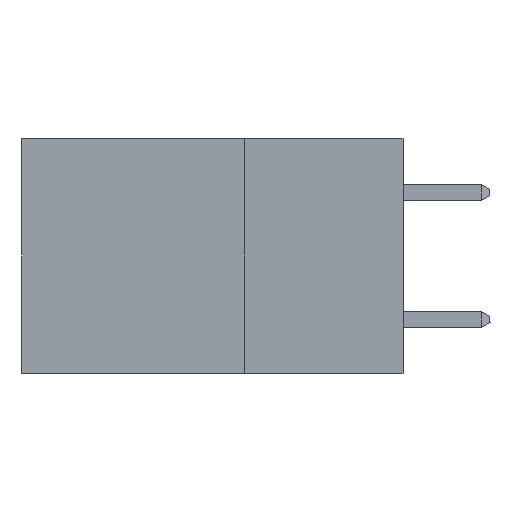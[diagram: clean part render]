
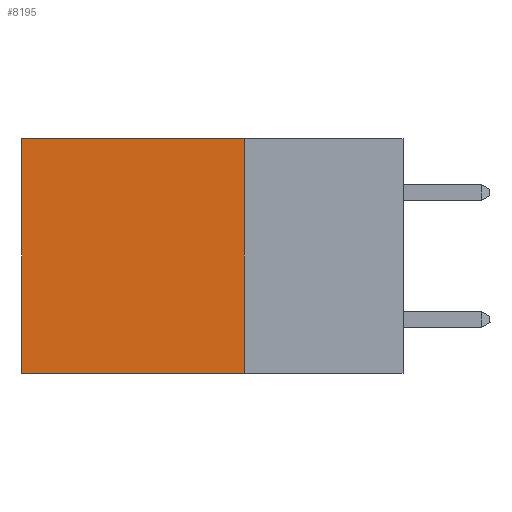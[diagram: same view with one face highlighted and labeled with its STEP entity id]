
A CAD part, left-side view. The second image highlights one B-rep face of the part: STEP entity #8195.
In plain terms, the highlighted planar face has unit normal (-1, 0, 0).
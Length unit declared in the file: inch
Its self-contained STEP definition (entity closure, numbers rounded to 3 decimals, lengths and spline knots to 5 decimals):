
#288 = LINE ( 'NONE', #4807, #12843 ) ;
#349 = CARTESIAN_POINT ( 'NONE',  ( 0.2875, 0.25, 0. ) ) ;
#1516 = DIRECTION ( 'NONE',  ( 0., 0., -1. ) ) ;
#1641 = LINE ( 'NONE', #9368, #4037 ) ;
#2207 = CARTESIAN_POINT ( 'NONE',  ( 0.2875, 0.25, 0. ) ) ;
#2463 = EDGE_CURVE ( 'NONE', #10971, #2933, #1641, .T. ) ;
#2933 = VERTEX_POINT ( 'NONE', #4851 ) ;
#3412 = DIRECTION ( 'NONE',  ( 1., 0., 0. ) ) ;
#3522 = FACE_OUTER_BOUND ( 'NONE', #11455, .T. ) ;
#4037 = VECTOR ( 'NONE', #1516, 39.37008 ) ;
#4088 = VERTEX_POINT ( 'NONE', #11445 ) ;
#4428 = LINE ( 'NONE', #11561, #7418 ) ;
#4807 = CARTESIAN_POINT ( 'NONE',  ( 0.2875, 0.25, -0.37 ) ) ;
#4851 = CARTESIAN_POINT ( 'NONE',  ( 0.2875, 0.25, -0.37 ) ) ;
#6516 = ORIENTED_EDGE ( 'NONE', *, *, #8967, .T. ) ;
#6589 = DIRECTION ( 'NONE',  ( 0., 0., -1. ) ) ;
#7290 = AXIS2_PLACEMENT_3D ( 'NONE', #2207, #3412, #12049 ) ;
#7418 = VECTOR ( 'NONE', #6589, 39.37008 ) ;
#7448 = CARTESIAN_POINT ( 'NONE',  ( 0.2875, 0.25, 0. ) ) ;
#7703 = LINE ( 'NONE', #349, #13649 ) ;
#8193 = ORIENTED_EDGE ( 'NONE', *, *, #9516, .F. ) ;
#8195 = ADVANCED_FACE ( 'NONE', ( #3522 ), #9686, .F. ) ;
#8201 = CARTESIAN_POINT ( 'NONE',  ( 0.2875, 0.6, 0. ) ) ;
#8801 = ORIENTED_EDGE ( 'NONE', *, *, #2463, .F. ) ;
#8962 = DIRECTION ( 'NONE',  ( 0., 1., 0. ) ) ;
#8967 = EDGE_CURVE ( 'NONE', #12378, #4088, #4428, .T. ) ;
#9130 = ORIENTED_EDGE ( 'NONE', *, *, #14373, .T. ) ;
#9368 = CARTESIAN_POINT ( 'NONE',  ( 0.2875, 0.25, 0. ) ) ;
#9516 = EDGE_CURVE ( 'NONE', #2933, #4088, #288, .T. ) ;
#9686 = PLANE ( 'NONE',  #7290 ) ;
#10971 = VERTEX_POINT ( 'NONE', #7448 ) ;
#11445 = CARTESIAN_POINT ( 'NONE',  ( 0.2875, 0.6, -0.37 ) ) ;
#11455 = EDGE_LOOP ( 'NONE', ( #6516, #8193, #8801, #9130 ) ) ;
#11561 = CARTESIAN_POINT ( 'NONE',  ( 0.2875, 0.6, 0. ) ) ;
#12049 = DIRECTION ( 'NONE',  ( 0., 0., -1. ) ) ;
#12242 = DIRECTION ( 'NONE',  ( 0., 1., 0. ) ) ;
#12378 = VERTEX_POINT ( 'NONE', #8201 ) ;
#12843 = VECTOR ( 'NONE', #12242, 39.37008 ) ;
#13649 = VECTOR ( 'NONE', #8962, 39.37008 ) ;
#14373 = EDGE_CURVE ( 'NONE', #10971, #12378, #7703, .T. ) ;
